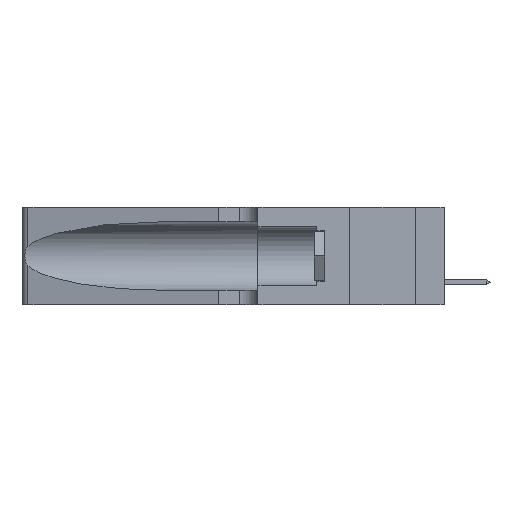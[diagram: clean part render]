
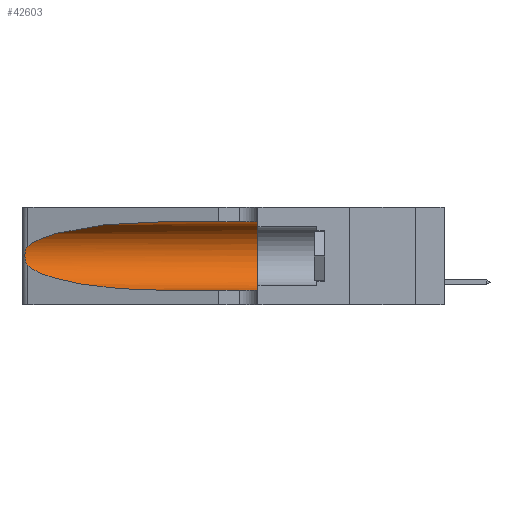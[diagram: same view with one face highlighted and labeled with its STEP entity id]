
A CAD part, left-side view. The second image highlights one B-rep face of the part: STEP entity #42603.
In plain terms, the highlighted cylindrical face has radius 3.308 mm (diameter 6.617 mm), a partial arc.
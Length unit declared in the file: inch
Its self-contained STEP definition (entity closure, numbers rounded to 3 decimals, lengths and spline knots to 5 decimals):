
#74 =( BOUNDED_CURVE ( )  B_SPLINE_CURVE ( 3, ( #36050, #9611, #39718, #5957 ),
 .UNSPECIFIED., .F., .F. ) 
 B_SPLINE_CURVE_WITH_KNOTS ( ( 4, 4 ),
 ( 1.5708, 2.84003 ),
 .UNSPECIFIED. ) 
 CURVE ( )  GEOMETRIC_REPRESENTATION_ITEM ( )  RATIONAL_B_SPLINE_CURVE ( ( 1., 0.87, 0.87, 1. ) ) 
 REPRESENTATION_ITEM ( '' )  );
#2752 = EDGE_CURVE ( 'NONE', #36358, #11428, #13193, .T. ) ;
#2797 = VERTEX_POINT ( 'NONE', #18986 ) ;
#4374 = DIRECTION ( 'NONE',  ( 0., -1., 0. ) ) ;
#4611 = CARTESIAN_POINT ( 'NONE',  ( 0.26018, 1.23835, 0.19895 ) ) ;
#5957 = CARTESIAN_POINT ( 'NONE',  ( 0.25487, 1.22718, 0.22369 ) ) ;
#7046 = DIRECTION ( 'NONE',  ( 0., -1., 0. ) ) ;
#8118 = FACE_OUTER_BOUND ( 'NONE', #38684, .T. ) ;
#8144 = CARTESIAN_POINT ( 'NONE',  ( 0.26075, 1.23896, 0.19203 ) ) ;
#8294 = CARTESIAN_POINT ( 'NONE',  ( 0.25639, 1.23186, 0.15144 ) ) ;
#8770 = LINE ( 'NONE', #24182, #26982 ) ;
#9468 = CARTESIAN_POINT ( 'NONE',  ( 0.1305, 0.72297, 0.31525 ) ) ;
#9611 = CARTESIAN_POINT ( 'NONE',  ( 0.18966, 0.96281, 0.31525 ) ) ;
#10696 = CARTESIAN_POINT ( 'NONE',  ( 0.1305, 1.61858, 0.05475 ) ) ;
#11207 = CARTESIAN_POINT ( 'NONE',  ( 0.25639, 1.23184, 0.21858 ) ) ;
#11428 = VERTEX_POINT ( 'NONE', #18536 ) ;
#12056 = CARTESIAN_POINT ( 'NONE',  ( 0.1305, 0.35, 0.05475 ) ) ;
#13193 =( BOUNDED_CURVE ( )  B_SPLINE_CURVE ( 3, ( #42516, #35790, #35651, #29199 ),
 .UNSPECIFIED., .F., .T. ) 
 B_SPLINE_CURVE_WITH_KNOTS ( ( 4, 4 ),
 ( 3.44316, 4.71239 ),
 .UNSPECIFIED. ) 
 CURVE ( )  GEOMETRIC_REPRESENTATION_ITEM ( )  RATIONAL_B_SPLINE_CURVE ( ( 1., 0.87, 0.87, 1. ) ) 
 REPRESENTATION_ITEM ( '' )  );
#15604 = AXIS2_PLACEMENT_3D ( 'NONE', #41648, #4374, #38149 ) ;
#15957 = LINE ( 'NONE', #10696, #28457 ) ;
#16113 = ORIENTED_EDGE ( 'NONE', *, *, #42414, .T. ) ;
#16293 = AXIS2_PLACEMENT_3D ( 'NONE', #21978, #38965, #35411 ) ;
#17110 = ORIENTED_EDGE ( 'NONE', *, *, #2752, .T. ) ;
#17596 = CARTESIAN_POINT ( 'NONE',  ( 0.25787, 1.23484, 0.2124 ) ) ;
#17891 = ORIENTED_EDGE ( 'NONE', *, *, #41727, .F. ) ;
#17892 = CARTESIAN_POINT ( 'NONE',  ( 0.25854, 1.2359, 0.20912 ) ) ;
#18480 = CARTESIAN_POINT ( 'NONE',  ( 0.25856, 1.23593, 0.16098 ) ) ;
#18536 = CARTESIAN_POINT ( 'NONE',  ( 0.1305, 0.72297, 0.05475 ) ) ;
#18986 = CARTESIAN_POINT ( 'NONE',  ( 0.1305, 0.35, 0.31525 ) ) ;
#20537 = DIRECTION ( 'NONE',  ( 0., -1., 0. ) ) ;
#21866 = CARTESIAN_POINT ( 'NONE',  ( 0.25487, 1.22718, 0.14631 ) ) ;
#21978 = CARTESIAN_POINT ( 'NONE',  ( 0.1305, 0.35, 0.185 ) ) ;
#24182 = CARTESIAN_POINT ( 'NONE',  ( 0.1305, 1.61858, 0.31525 ) ) ;
#24633 = CARTESIAN_POINT ( 'NONE',  ( 0.25555, 1.22994, 0.2215 ) ) ;
#24689 = B_SPLINE_CURVE_WITH_KNOTS ( 'NONE', 3,
 ( #30907, #24633, #11207, #17596, #17892, #4611, #8144, #35455, #42028, #18480, #41731, #8294, #25218, #21866 ),
 .UNSPECIFIED., .F., .F.,
 ( 4, 2, 2, 2, 2, 2, 4 ),
 ( 0., 0.00027, 0.00053, 0.00107, 0.0016, 0.00187, 0.00214 ),
 .UNSPECIFIED. ) ;
#25218 = CARTESIAN_POINT ( 'NONE',  ( 0.25555, 1.22993, 0.14849 ) ) ;
#25671 = ORIENTED_EDGE ( 'NONE', *, *, #34095, .T. ) ;
#26899 = CYLINDRICAL_SURFACE ( 'NONE', #15604, 0.13025 ) ;
#26982 = VECTOR ( 'NONE', #20537, 39.37008 ) ;
#27442 = CIRCLE ( 'NONE', #16293, 0.13025 ) ;
#28137 = CARTESIAN_POINT ( 'NONE',  ( 0.25487, 1.22718, 0.14631 ) ) ;
#28457 = VECTOR ( 'NONE', #7046, 39.37008 ) ;
#28830 = EDGE_CURVE ( 'NONE', #34363, #33285, #74, .T. ) ;
#29199 = CARTESIAN_POINT ( 'NONE',  ( 0.1305, 0.72297, 0.05475 ) ) ;
#29676 = ORIENTED_EDGE ( 'NONE', *, *, #36897, .F. ) ;
#30907 = CARTESIAN_POINT ( 'NONE',  ( 0.25487, 1.22718, 0.22369 ) ) ;
#32995 = VERTEX_POINT ( 'NONE', #12056 ) ;
#33285 = VERTEX_POINT ( 'NONE', #40594 ) ;
#34095 = EDGE_CURVE ( 'NONE', #33285, #36358, #24689, .T. ) ;
#34363 = VERTEX_POINT ( 'NONE', #9468 ) ;
#35411 = DIRECTION ( 'NONE',  ( 0., 0., 1. ) ) ;
#35455 = CARTESIAN_POINT ( 'NONE',  ( 0.26075, 1.23896, 0.178 ) ) ;
#35651 = CARTESIAN_POINT ( 'NONE',  ( 0.18966, 0.96281, 0.05475 ) ) ;
#35790 = CARTESIAN_POINT ( 'NONE',  ( 0.2373, 1.15595, 0.08982 ) ) ;
#36050 = CARTESIAN_POINT ( 'NONE',  ( 0.1305, 0.72297, 0.31525 ) ) ;
#36358 = VERTEX_POINT ( 'NONE', #28137 ) ;
#36897 = EDGE_CURVE ( 'NONE', #2797, #32995, #27442, .T. ) ;
#38149 = DIRECTION ( 'NONE',  ( 0., 0., -1. ) ) ;
#38684 = EDGE_LOOP ( 'NONE', ( #41453, #25671, #17110, #16113, #29676, #17891 ) ) ;
#38965 = DIRECTION ( 'NONE',  ( 0., 1., 0. ) ) ;
#39718 = CARTESIAN_POINT ( 'NONE',  ( 0.2373, 1.15595, 0.28018 ) ) ;
#40594 = CARTESIAN_POINT ( 'NONE',  ( 0.25487, 1.22718, 0.22369 ) ) ;
#41453 = ORIENTED_EDGE ( 'NONE', *, *, #28830, .T. ) ;
#41648 = CARTESIAN_POINT ( 'NONE',  ( 0.1305, 1.61858, 0.185 ) ) ;
#41727 = EDGE_CURVE ( 'NONE', #34363, #2797, #8770, .T. ) ;
#41731 = CARTESIAN_POINT ( 'NONE',  ( 0.25789, 1.23486, 0.15765 ) ) ;
#42028 = CARTESIAN_POINT ( 'NONE',  ( 0.26017, 1.23833, 0.17102 ) ) ;
#42414 = EDGE_CURVE ( 'NONE', #11428, #32995, #15957, .T. ) ;
#42516 = CARTESIAN_POINT ( 'NONE',  ( 0.25487, 1.22718, 0.14631 ) ) ;
#42603 = ADVANCED_FACE ( 'NONE', ( #8118 ), #26899, .F. ) ;
